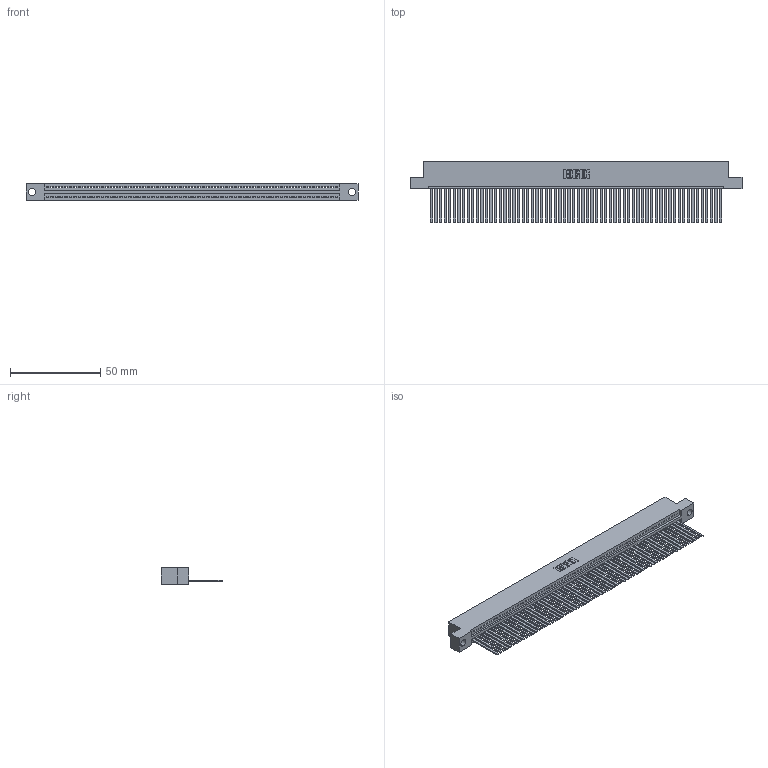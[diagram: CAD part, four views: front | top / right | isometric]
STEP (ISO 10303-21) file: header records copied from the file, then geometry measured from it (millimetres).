
FILE_DESCRIPTION (( 'STEP AP203' ), '1' );
FILE_NAME ('395-064-544-104.STEP', '2019-10-25T03:14:28', ( '' ), ( '' ), 'SwSTEP 2.0', 'SolidWorks 2016', '' );
FILE_SCHEMA (( 'CONFIG_CONTROL_DESIGN' ));
Length unit declared in the file: inch
Products named in the file (3): 345 Part_Flush Mounting Lugs - 0.156 Dia-TH; 395-064-544-104; 345-292-001_345-293-144
Assembly tree (65 placements, depth 2):
  395-064-544-104
    345 Part_Flush Mounting Lugs - 0.156 Dia-TH
    345-292-001_345-293-144  x64
Bounding box: 183.77 x 33.96 x 9.4 mm (x, y, z)
Volume: 18288.1 mm3; surface area: 26636.2 mm2
Topology: 65 solids, 65 shells, 3454 faces, 10453 edges, 6882 vertices
Faces by surface type: plane 2384, cylinder 1070
Entity records: 45025 total; most frequent: CARTESIAN_POINT 7804, ORIENTED_EDGE 7802, DIRECTION 6781, EDGE_CURVE 3901, VECTOR 3517, LINE 3517, VERTEX_POINT 2598, AXIS2_PLACEMENT_3D 1632
